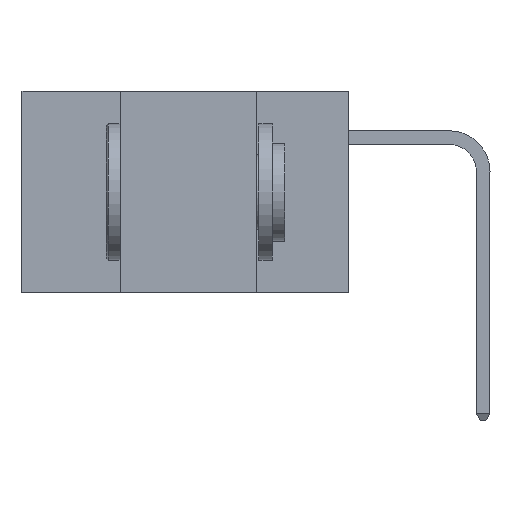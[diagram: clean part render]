
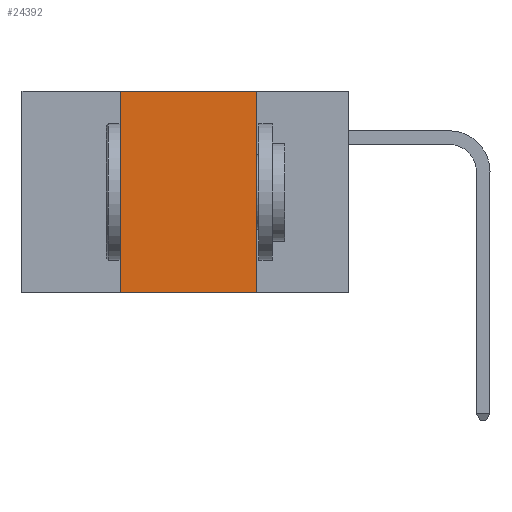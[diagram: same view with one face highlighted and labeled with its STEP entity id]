
A CAD part, left-side view. The second image highlights one B-rep face of the part: STEP entity #24392.
In plain terms, the highlighted planar face has unit normal (-1, 0, 0).
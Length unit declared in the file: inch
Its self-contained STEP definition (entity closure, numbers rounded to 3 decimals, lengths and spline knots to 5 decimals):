
#1197 = EDGE_CURVE ( 'NONE', #30734, #19151, #32779, .T. ) ;
#3007 = CARTESIAN_POINT ( 'NONE',  ( 0., 0.6, 0. ) ) ;
#5605 = EDGE_CURVE ( 'NONE', #24442, #30734, #25943, .T. ) ;
#8262 = LINE ( 'NONE', #20224, #28262 ) ;
#8746 = DIRECTION ( 'NONE',  ( 0., 0., 1. ) ) ;
#9715 = EDGE_LOOP ( 'NONE', ( #27085, #27465, #27906, #28011 ) ) ;
#9931 = DIRECTION ( 'NONE',  ( 0., -1., 0. ) ) ;
#10356 = VECTOR ( 'NONE', #10809, 39.37008 ) ;
#10809 = DIRECTION ( 'NONE',  ( 0., 0., -1. ) ) ;
#10817 = VECTOR ( 'NONE', #34847, 39.37008 ) ;
#10856 = CARTESIAN_POINT ( 'NONE',  ( 0., 0.42, -0.37 ) ) ;
#13350 = LINE ( 'NONE', #32428, #16555 ) ;
#13539 = CARTESIAN_POINT ( 'NONE',  ( 0., 0.17, 0. ) ) ;
#14874 = DIRECTION ( 'NONE',  ( 1., 0., 0. ) ) ;
#15141 = CARTESIAN_POINT ( 'NONE',  ( 0., 0.42, 0. ) ) ;
#15495 = VERTEX_POINT ( 'NONE', #10856 ) ;
#16555 = VECTOR ( 'NONE', #9931, 39.37008 ) ;
#17899 = CARTESIAN_POINT ( 'NONE',  ( 0., 0.17, -0.37 ) ) ;
#19151 = VERTEX_POINT ( 'NONE', #17899 ) ;
#20224 = CARTESIAN_POINT ( 'NONE',  ( 0., 0.42, 0. ) ) ;
#23965 = CARTESIAN_POINT ( 'NONE',  ( 0., 0.6, 0. ) ) ;
#24392 = ADVANCED_FACE ( 'NONE', ( #31807 ), #31640, .F. ) ;
#24442 = VERTEX_POINT ( 'NONE', #15141 ) ;
#25581 = CARTESIAN_POINT ( 'NONE',  ( 0., 0.17, 0. ) ) ;
#25943 = LINE ( 'NONE', #23965, #10817 ) ;
#27085 = ORIENTED_EDGE ( 'NONE', *, *, #1197, .F. ) ;
#27465 = ORIENTED_EDGE ( 'NONE', *, *, #5605, .F. ) ;
#27906 = ORIENTED_EDGE ( 'NONE', *, *, #30830, .F. ) ;
#28011 = ORIENTED_EDGE ( 'NONE', *, *, #29017, .T. ) ;
#28262 = VECTOR ( 'NONE', #8746, 39.37008 ) ;
#29017 = EDGE_CURVE ( 'NONE', #15495, #19151, #13350, .T. ) ;
#29360 = AXIS2_PLACEMENT_3D ( 'NONE', #3007, #14874, #34366 ) ;
#30734 = VERTEX_POINT ( 'NONE', #25581 ) ;
#30830 = EDGE_CURVE ( 'NONE', #15495, #24442, #8262, .T. ) ;
#31640 = PLANE ( 'NONE',  #29360 ) ;
#31807 = FACE_OUTER_BOUND ( 'NONE', #9715, .T. ) ;
#32428 = CARTESIAN_POINT ( 'NONE',  ( 0., 0.6, -0.37 ) ) ;
#32779 = LINE ( 'NONE', #13539, #10356 ) ;
#34366 = DIRECTION ( 'NONE',  ( 0., 0., -1. ) ) ;
#34847 = DIRECTION ( 'NONE',  ( 0., -1., 0. ) ) ;
